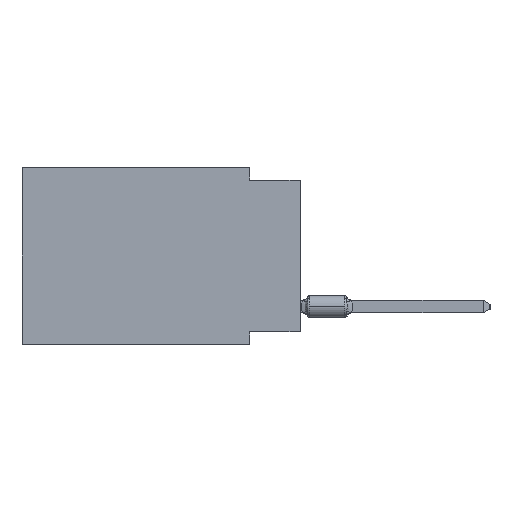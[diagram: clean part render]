
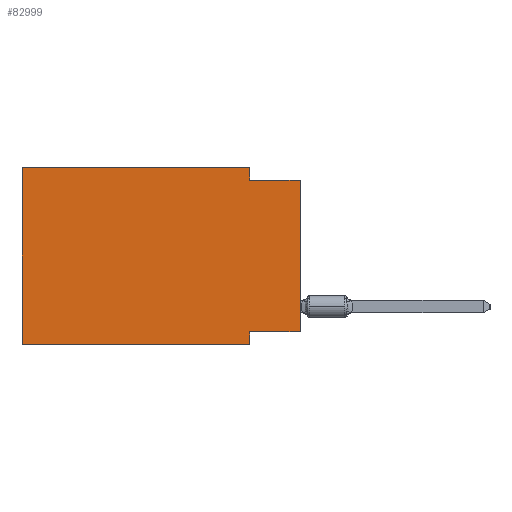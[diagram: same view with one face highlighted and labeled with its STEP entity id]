
A CAD part, left-side view. The second image highlights one B-rep face of the part: STEP entity #82999.
In plain terms, the highlighted planar face has unit normal (-1, 0, 0).
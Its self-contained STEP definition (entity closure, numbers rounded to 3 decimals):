
#2140 = VERTEX_POINT ( 'NONE', #99219 ) ;
#2407 = EDGE_CURVE ( 'NONE', #37947, #109676, #54052, .T. ) ;
#3662 = VECTOR ( 'NONE', #88043, 1000. ) ;
#6591 = DIRECTION ( 'NONE',  ( 0., 0., 1. ) ) ;
#7901 = CARTESIAN_POINT ( 'NONE',  ( 0., 2.54, -0.635 ) ) ;
#8719 = CARTESIAN_POINT ( 'NONE',  ( 0., 0., -8.255 ) ) ;
#11664 = CARTESIAN_POINT ( 'NONE',  ( 0., 0., -0.635 ) ) ;
#12358 = VECTOR ( 'NONE', #25073, 1000. ) ;
#13892 = CARTESIAN_POINT ( 'NONE',  ( 0., 13.97, 0. ) ) ;
#15259 = ORIENTED_EDGE ( 'NONE', *, *, #20274, .F. ) ;
#16982 = VECTOR ( 'NONE', #37322, 1000. ) ;
#20024 = ORIENTED_EDGE ( 'NONE', *, *, #70373, .F. ) ;
#20274 = EDGE_CURVE ( 'NONE', #109016, #106340, #32590, .T. ) ;
#25073 = DIRECTION ( 'NONE',  ( 0., -1., 0. ) ) ;
#27381 = AXIS2_PLACEMENT_3D ( 'NONE', #13892, #57951, #32287 ) ;
#27891 = ORIENTED_EDGE ( 'NONE', *, *, #74173, .T. ) ;
#30572 = CARTESIAN_POINT ( 'NONE',  ( 0., 13.97, 0. ) ) ;
#32287 = DIRECTION ( 'NONE',  ( 0., 0., -1. ) ) ;
#32590 = LINE ( 'NONE', #66030, #48678 ) ;
#33819 = LINE ( 'NONE', #8719, #98564 ) ;
#37322 = DIRECTION ( 'NONE',  ( 0., -1., 0. ) ) ;
#37947 = VERTEX_POINT ( 'NONE', #7901 ) ;
#38413 = LINE ( 'NONE', #30572, #41112 ) ;
#39349 = ORIENTED_EDGE ( 'NONE', *, *, #99007, .F. ) ;
#40563 = CARTESIAN_POINT ( 'NONE',  ( 0., 2.54, -8.89 ) ) ;
#41112 = VECTOR ( 'NONE', #6591, 1000. ) ;
#41115 = ORIENTED_EDGE ( 'NONE', *, *, #105888, .F. ) ;
#42900 = CARTESIAN_POINT ( 'NONE',  ( 0., 13.97, 0. ) ) ;
#44541 = VERTEX_POINT ( 'NONE', #52491 ) ;
#47233 = EDGE_CURVE ( 'NONE', #44541, #106340, #60951, .T. ) ;
#48678 = VECTOR ( 'NONE', #91650, 1000. ) ;
#49034 = PLANE ( 'NONE',  #27381 ) ;
#52491 = CARTESIAN_POINT ( 'NONE',  ( 0., 13.97, -8.89 ) ) ;
#52588 = CARTESIAN_POINT ( 'NONE',  ( 0., 13.97, -8.89 ) ) ;
#53822 = CARTESIAN_POINT ( 'NONE',  ( 0., 13.97, 0. ) ) ;
#54052 = LINE ( 'NONE', #11664, #16982 ) ;
#54319 = DIRECTION ( 'NONE',  ( 0., 0., 1. ) ) ;
#56290 = FACE_OUTER_BOUND ( 'NONE', #107659, .T. ) ;
#56798 = ORIENTED_EDGE ( 'NONE', *, *, #2407, .F. ) ;
#57881 = CARTESIAN_POINT ( 'NONE',  ( 0., 0., -0.635 ) ) ;
#57951 = DIRECTION ( 'NONE',  ( 1., 0., 0. ) ) ;
#59312 = EDGE_CURVE ( 'NONE', #44541, #72292, #38413, .T. ) ;
#60951 = LINE ( 'NONE', #52588, #3662 ) ;
#61985 = VECTOR ( 'NONE', #101552, 1000. ) ;
#64944 = ORIENTED_EDGE ( 'NONE', *, *, #59312, .F. ) ;
#66030 = CARTESIAN_POINT ( 'NONE',  ( 0., 2.54, -8.89 ) ) ;
#66162 = VECTOR ( 'NONE', #54319, 1000. ) ;
#67572 = LINE ( 'NONE', #100992, #61985 ) ;
#67813 = DIRECTION ( 'NONE',  ( 0., 1., 0. ) ) ;
#69929 = LINE ( 'NONE', #103361, #66162 ) ;
#70373 = EDGE_CURVE ( 'NONE', #2140, #37947, #67572, .T. ) ;
#72292 = VERTEX_POINT ( 'NONE', #53822 ) ;
#74173 = EDGE_CURVE ( 'NONE', #86006, #109676, #69929, .T. ) ;
#82999 = ADVANCED_FACE ( 'NONE', ( #56290 ), #49034, .F. ) ;
#84700 = LINE ( 'NONE', #42900, #12358 ) ;
#86006 = VERTEX_POINT ( 'NONE', #98926 ) ;
#88043 = DIRECTION ( 'NONE',  ( 0., -1., 0. ) ) ;
#88746 = CARTESIAN_POINT ( 'NONE',  ( 0., 2.54, -8.255 ) ) ;
#91650 = DIRECTION ( 'NONE',  ( 0., 0., -1. ) ) ;
#92550 = ORIENTED_EDGE ( 'NONE', *, *, #47233, .T. ) ;
#98564 = VECTOR ( 'NONE', #67813, 1000. ) ;
#98926 = CARTESIAN_POINT ( 'NONE',  ( 0., 0., -8.255 ) ) ;
#99007 = EDGE_CURVE ( 'NONE', #86006, #109016, #33819, .T. ) ;
#99219 = CARTESIAN_POINT ( 'NONE',  ( 0., 2.54, 0. ) ) ;
#100992 = CARTESIAN_POINT ( 'NONE',  ( 0., 2.54, 0. ) ) ;
#101552 = DIRECTION ( 'NONE',  ( 0., 0., -1. ) ) ;
#103361 = CARTESIAN_POINT ( 'NONE',  ( 0., 0., 0. ) ) ;
#105888 = EDGE_CURVE ( 'NONE', #72292, #2140, #84700, .T. ) ;
#106340 = VERTEX_POINT ( 'NONE', #40563 ) ;
#107659 = EDGE_LOOP ( 'NONE', ( #27891, #56798, #20024, #41115, #64944, #92550, #15259, #39349 ) ) ;
#109016 = VERTEX_POINT ( 'NONE', #88746 ) ;
#109676 = VERTEX_POINT ( 'NONE', #57881 ) ;
